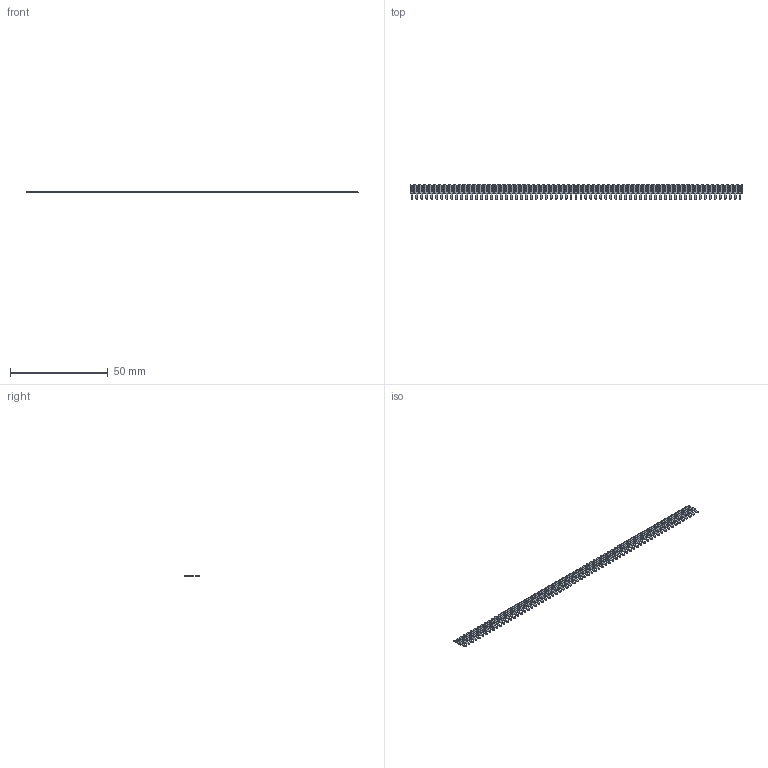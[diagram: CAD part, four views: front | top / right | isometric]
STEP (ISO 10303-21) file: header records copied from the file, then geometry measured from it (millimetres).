
FILE_DESCRIPTION (( 'STEP AP203' ), '1' );
FILE_NAME ('103-067-253-100.STEP', '2020-04-16T16:42:02', ( '' ), ( '' ), 'SwSTEP 2.0', 'SolidWorks 2016', '' );
FILE_SCHEMA (( 'CONFIG_CONTROL_DESIGN' ));
Length unit declared in the file: inch
Products named in the file (2): 103-067-253-100; 100-290-001_100-290-253
Assembly tree (67 placements, depth 2):
  103-067-253-100
    100-290-001_100-290-253  x67
Bounding box: 169.67 x 7.62 x 0.51 mm (x, y, z)
Volume: 369.7 mm3; surface area: 2305.3 mm2
Topology: 67 solids, 67 shells, 1340 faces, 3618 edges, 2412 vertices
Faces by surface type: plane 1273, cylinder 67
Entity records: 2932 total; most frequent: DIRECTION 236, CARTESIAN_POINT 180, DATE_AND_TIME 144, COORDINATED_UNIVERSAL_TIME_OFFSET 144, CALENDAR_DATE 144, LOCAL_TIME 144, ORIENTED_EDGE 108, AXIS2_PLACEMENT_3D 92
